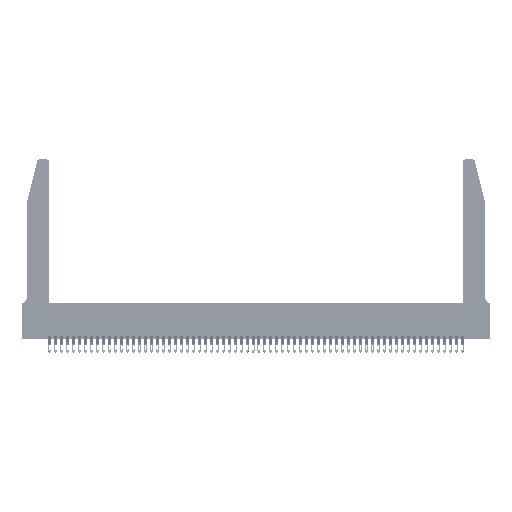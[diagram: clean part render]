
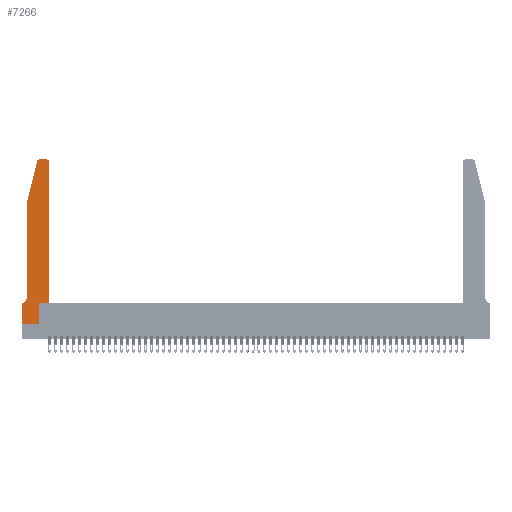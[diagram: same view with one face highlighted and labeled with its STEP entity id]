
A CAD part, top view. The second image highlights one B-rep face of the part: STEP entity #7266.
In plain terms, the highlighted planar face has unit normal (0, 0, 1).
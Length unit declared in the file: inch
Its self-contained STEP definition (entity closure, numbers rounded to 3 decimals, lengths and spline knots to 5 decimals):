
#190 = VERTEX_POINT ( 'NONE', #19763 ) ;
#552 = EDGE_CURVE ( 'NONE', #43524, #5490, #48906, .T. ) ;
#1331 = ORIENTED_EDGE ( 'NONE', *, *, #36567, .T. ) ;
#1723 = AXIS2_PLACEMENT_3D ( 'NONE', #37468, #28571, #38035 ) ;
#3138 = ORIENTED_EDGE ( 'NONE', *, *, #54369, .T. ) ;
#3342 = VECTOR ( 'NONE', #33266, 39.37008 ) ;
#4205 = EDGE_CURVE ( 'NONE', #12866, #27678, #9803, .T. ) ;
#4374 = CIRCLE ( 'NONE', #16417, 0.03 ) ;
#5198 = ORIENTED_EDGE ( 'NONE', *, *, #552, .T. ) ;
#5284 = EDGE_CURVE ( 'NONE', #18872, #35536, #26629, .T. ) ;
#5490 = VERTEX_POINT ( 'NONE', #11655 ) ;
#5804 = LINE ( 'NONE', #40007, #25522 ) ;
#6710 = LINE ( 'NONE', #50050, #31166 ) ;
#7060 = CARTESIAN_POINT ( 'NONE',  ( 0.0755, 0.35, 0.37 ) ) ;
#7266 = ADVANCED_FACE ( 'NONE', ( #43648 ), #49441, .T. ) ;
#7521 = CARTESIAN_POINT ( 'NONE',  ( 0.0755, 2., 0.37 ) ) ;
#8013 = DIRECTION ( 'NONE',  ( 1., 0., 0. ) ) ;
#8208 = CARTESIAN_POINT ( 'NONE',  ( 0.2865, 0.35, 0.37 ) ) ;
#9803 = LINE ( 'NONE', #7521, #18607 ) ;
#9833 = VERTEX_POINT ( 'NONE', #36971 ) ;
#11096 = DIRECTION ( 'NONE',  ( 1., 0., 0. ) ) ;
#11655 = CARTESIAN_POINT ( 'NONE',  ( 0.4505, 2.72, 0.37 ) ) ;
#11796 = ORIENTED_EDGE ( 'NONE', *, *, #18499, .T. ) ;
#11985 = DIRECTION ( 'NONE',  ( 0., 0., 1. ) ) ;
#12866 = VERTEX_POINT ( 'NONE', #36411 ) ;
#13949 = VERTEX_POINT ( 'NONE', #40098 ) ;
#14111 = CARTESIAN_POINT ( 'NONE',  ( 0., 0., 0.37 ) ) ;
#14211 = VECTOR ( 'NONE', #30146, 39.37008 ) ;
#14256 = CARTESIAN_POINT ( 'NONE',  ( 0., 0., 0.37 ) ) ;
#14871 = VERTEX_POINT ( 'NONE', #26193 ) ;
#15494 = LINE ( 'NONE', #7060, #3342 ) ;
#15937 = ORIENTED_EDGE ( 'NONE', *, *, #20193, .T. ) ;
#16417 = AXIS2_PLACEMENT_3D ( 'NONE', #16689, #11985, #8013 ) ;
#16561 = DIRECTION ( 'NONE',  ( 0., -1., 0. ) ) ;
#16689 = CARTESIAN_POINT ( 'NONE',  ( 0.4205, 2.72, 0.37 ) ) ;
#18126 = CARTESIAN_POINT ( 'NONE',  ( 0.0055, 0.42, 0.37 ) ) ;
#18300 = DIRECTION ( 'NONE',  ( 0., 0., 1. ) ) ;
#18499 = EDGE_CURVE ( 'NONE', #41944, #18872, #6710, .T. ) ;
#18607 = VECTOR ( 'NONE', #33343, 39.37008 ) ;
#18872 = VERTEX_POINT ( 'NONE', #14256 ) ;
#19763 = CARTESIAN_POINT ( 'NONE',  ( 0.0755, 0.42, 0.37 ) ) ;
#20193 = EDGE_CURVE ( 'NONE', #14871, #9833, #24169, .T. ) ;
#22965 = LINE ( 'NONE', #38293, #48055 ) ;
#24169 = LINE ( 'NONE', #44148, #41160 ) ;
#24992 = ORIENTED_EDGE ( 'NONE', *, *, #33745, .T. ) ;
#25522 = VECTOR ( 'NONE', #27072, 39.37008 ) ;
#25665 = DIRECTION ( 'NONE',  ( 0., 1., 0. ) ) ;
#26193 = CARTESIAN_POINT ( 'NONE',  ( 0.4205, 2.75, 0.37 ) ) ;
#26629 = LINE ( 'NONE', #14111, #40271 ) ;
#27022 = CARTESIAN_POINT ( 'NONE',  ( 0.0755, 2., 0.37 ) ) ;
#27072 = DIRECTION ( 'NONE',  ( 1., 0., 0. ) ) ;
#27678 = VERTEX_POINT ( 'NONE', #27022 ) ;
#28130 = VECTOR ( 'NONE', #25665, 39.37008 ) ;
#28221 = CIRCLE ( 'NONE', #35585, 0.07 ) ;
#28571 = DIRECTION ( 'NONE',  ( 0., 0., 1. ) ) ;
#30146 = DIRECTION ( 'NONE',  ( 0., 1., 0. ) ) ;
#30277 = AXIS2_PLACEMENT_3D ( 'NONE', #49239, #18300, #31791 ) ;
#30675 = DIRECTION ( 'NONE',  ( 0., 0., -1. ) ) ;
#31166 = VECTOR ( 'NONE', #16561, 39.37008 ) ;
#31791 = DIRECTION ( 'NONE',  ( 1., 0., 0. ) ) ;
#32006 = ORIENTED_EDGE ( 'NONE', *, *, #55287, .T. ) ;
#33266 = DIRECTION ( 'NONE',  ( -1., 0., 0. ) ) ;
#33343 = DIRECTION ( 'NONE',  ( -0.239, -0.971, 0. ) ) ;
#33745 = EDGE_CURVE ( 'NONE', #35536, #40153, #47119, .T. ) ;
#34404 = ORIENTED_EDGE ( 'NONE', *, *, #5284, .T. ) ;
#34416 = CARTESIAN_POINT ( 'NONE',  ( 0.2865, 0., 0.37 ) ) ;
#35536 = VERTEX_POINT ( 'NONE', #34416 ) ;
#35585 = AXIS2_PLACEMENT_3D ( 'NONE', #18126, #30675, #43753 ) ;
#35825 = DIRECTION ( 'NONE',  ( -1., 0., 0. ) ) ;
#36411 = CARTESIAN_POINT ( 'NONE',  ( 0.25487, 2.72718, 0.37 ) ) ;
#36567 = EDGE_CURVE ( 'NONE', #13949, #41944, #15494, .T. ) ;
#36971 = CARTESIAN_POINT ( 'NONE',  ( 0.284, 2.75, 0.37 ) ) ;
#37314 = EDGE_CURVE ( 'NONE', #27678, #190, #22965, .T. ) ;
#37389 = ORIENTED_EDGE ( 'NONE', *, *, #51455, .T. ) ;
#37468 = CARTESIAN_POINT ( 'NONE',  ( 0.284, 2.72, 0.37 ) ) ;
#37535 = DIRECTION ( 'NONE',  ( 0., -1., 0. ) ) ;
#38035 = DIRECTION ( 'NONE',  ( 1., 0., 0. ) ) ;
#38293 = CARTESIAN_POINT ( 'NONE',  ( 0.0755, 2., 0.37 ) ) ;
#38531 = CARTESIAN_POINT ( 'NONE',  ( 0.2865, 0.35, 0.37 ) ) ;
#39983 = CARTESIAN_POINT ( 'NONE',  ( 0.4505, 0.35, 0.37 ) ) ;
#40007 = CARTESIAN_POINT ( 'NONE',  ( 0.4505, 0.35, 0.37 ) ) ;
#40098 = CARTESIAN_POINT ( 'NONE',  ( 0.0055, 0.35, 0.37 ) ) ;
#40153 = VERTEX_POINT ( 'NONE', #38531 ) ;
#40271 = VECTOR ( 'NONE', #11096, 39.37008 ) ;
#40781 = CIRCLE ( 'NONE', #1723, 0.03 ) ;
#41160 = VECTOR ( 'NONE', #35825, 39.37008 ) ;
#41944 = VERTEX_POINT ( 'NONE', #42780 ) ;
#42100 = ORIENTED_EDGE ( 'NONE', *, *, #50609, .T. ) ;
#42780 = CARTESIAN_POINT ( 'NONE',  ( 0., 0.35, 0.37 ) ) ;
#43524 = VERTEX_POINT ( 'NONE', #39983 ) ;
#43648 = FACE_OUTER_BOUND ( 'NONE', #55496, .T. ) ;
#43753 = DIRECTION ( 'NONE',  ( -1., 0., 0. ) ) ;
#43774 = ORIENTED_EDGE ( 'NONE', *, *, #4205, .T. ) ;
#44148 = CARTESIAN_POINT ( 'NONE',  ( 0.2605, 2.75, 0.37 ) ) ;
#45814 = ORIENTED_EDGE ( 'NONE', *, *, #37314, .T. ) ;
#47119 = LINE ( 'NONE', #8208, #28130 ) ;
#48055 = VECTOR ( 'NONE', #37535, 39.37008 ) ;
#48906 = LINE ( 'NONE', #55607, #14211 ) ;
#49239 = CARTESIAN_POINT ( 'NONE',  ( 0., 0.35, 0.37 ) ) ;
#49441 = PLANE ( 'NONE',  #30277 ) ;
#50050 = CARTESIAN_POINT ( 'NONE',  ( 0., 0., 0.37 ) ) ;
#50609 = EDGE_CURVE ( 'NONE', #190, #13949, #28221, .T. ) ;
#51455 = EDGE_CURVE ( 'NONE', #9833, #12866, #40781, .T. ) ;
#54369 = EDGE_CURVE ( 'NONE', #40153, #43524, #5804, .T. ) ;
#55287 = EDGE_CURVE ( 'NONE', #5490, #14871, #4374, .T. ) ;
#55496 = EDGE_LOOP ( 'NONE', ( #15937, #37389, #43774, #45814, #42100, #1331, #11796, #34404, #24992, #3138, #5198, #32006 ) ) ;
#55607 = CARTESIAN_POINT ( 'NONE',  ( 0.4505, 0.35, 0.37 ) ) ;
